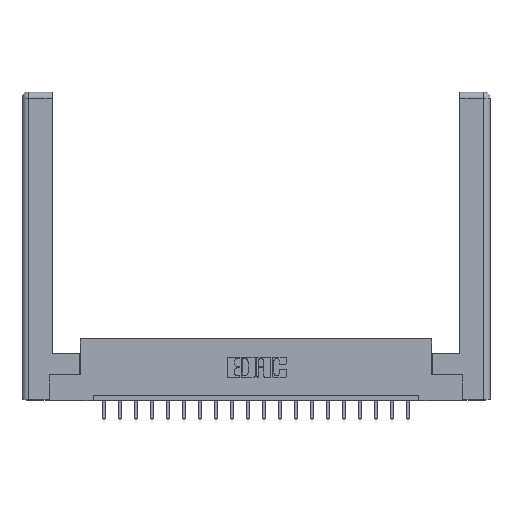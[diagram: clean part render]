
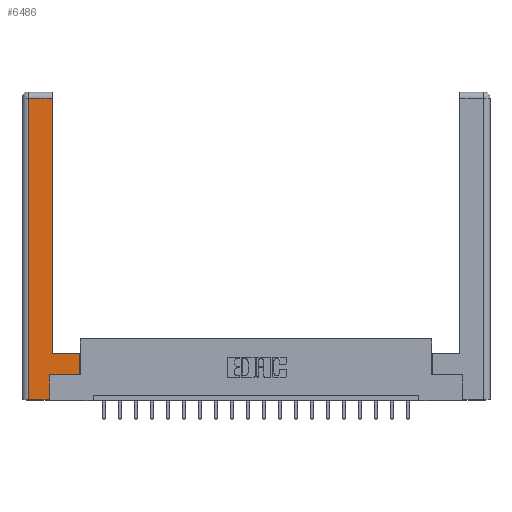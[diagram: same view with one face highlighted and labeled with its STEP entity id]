
A CAD part, top view. The second image highlights one B-rep face of the part: STEP entity #6486.
In plain terms, the highlighted planar face has unit normal (0, 0, 1).
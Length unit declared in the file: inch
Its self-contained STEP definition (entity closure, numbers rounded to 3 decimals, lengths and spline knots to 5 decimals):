
#60 = ORIENTED_EDGE ( 'NONE', *, *, #18326, .T. ) ;
#71 = PLANE ( 'NONE',  #1468 ) ;
#206 = ORIENTED_EDGE ( 'NONE', *, *, #640, .T. ) ;
#226 = DIRECTION ( 'NONE',  ( 0., -1., 0. ) ) ;
#282 = VECTOR ( 'NONE', #7637, 39.37008 ) ;
#640 = EDGE_CURVE ( 'NONE', #7224, #12169, #7378, .T. ) ;
#774 = CARTESIAN_POINT ( 'NONE',  ( 0.295, 2.94, 0. ) ) ;
#1060 = VERTEX_POINT ( 'NONE', #6679 ) ;
#1122 = VECTOR ( 'NONE', #226, 39.37008 ) ;
#1237 = CARTESIAN_POINT ( 'NONE',  ( 0.265, 0.245, 0. ) ) ;
#1468 = AXIS2_PLACEMENT_3D ( 'NONE', #14445, #1732, #1655 ) ;
#1655 = DIRECTION ( 'NONE',  ( -1., 0., 0. ) ) ;
#1732 = DIRECTION ( 'NONE',  ( 0., 0., -1. ) ) ;
#1901 = CARTESIAN_POINT ( 'NONE',  ( 0.565, 0.45, 0. ) ) ;
#1978 = EDGE_CURVE ( 'NONE', #12169, #1060, #11977, .T. ) ;
#2120 = LINE ( 'NONE', #3348, #1122 ) ;
#2153 = EDGE_CURVE ( 'NONE', #18739, #7224, #7045, .T. ) ;
#2240 = VERTEX_POINT ( 'NONE', #5527 ) ;
#2798 = VECTOR ( 'NONE', #3706, 39.37008 ) ;
#2805 = VECTOR ( 'NONE', #11432, 39.37008 ) ;
#3348 = CARTESIAN_POINT ( 'NONE',  ( 0.0615, 0., 0. ) ) ;
#3373 = ORIENTED_EDGE ( 'NONE', *, *, #14342, .T. ) ;
#3706 = DIRECTION ( 'NONE',  ( -1., 0., 0. ) ) ;
#3777 = LINE ( 'NONE', #5408, #11948 ) ;
#4193 = VERTEX_POINT ( 'NONE', #18626 ) ;
#4939 = EDGE_CURVE ( 'NONE', #2240, #4193, #10251, .T. ) ;
#5055 = VECTOR ( 'NONE', #6239, 39.37008 ) ;
#5352 = LINE ( 'NONE', #1901, #17923 ) ;
#5408 = CARTESIAN_POINT ( 'NONE',  ( 0.565, 0.245, 0. ) ) ;
#5441 = ORIENTED_EDGE ( 'NONE', *, *, #4939, .T. ) ;
#5527 = CARTESIAN_POINT ( 'NONE',  ( 0.0615, 0., 0. ) ) ;
#6239 = DIRECTION ( 'NONE',  ( -1., 0., 0. ) ) ;
#6486 = ADVANCED_FACE ( 'NONE', ( #15590 ), #71, .F. ) ;
#6679 = CARTESIAN_POINT ( 'NONE',  ( 0.0615, 2.94, 0. ) ) ;
#7045 = LINE ( 'NONE', #13186, #2798 ) ;
#7224 = VERTEX_POINT ( 'NONE', #16308 ) ;
#7378 = LINE ( 'NONE', #14216, #13511 ) ;
#7436 = CARTESIAN_POINT ( 'NONE',  ( 0.265, 0.245, 0. ) ) ;
#7622 = ORIENTED_EDGE ( 'NONE', *, *, #2153, .T. ) ;
#7637 = DIRECTION ( 'NONE',  ( 0., 1., 0. ) ) ;
#8750 = VERTEX_POINT ( 'NONE', #15575 ) ;
#10245 = ORIENTED_EDGE ( 'NONE', *, *, #14094, .T. ) ;
#10251 = LINE ( 'NONE', #14394, #2805 ) ;
#10887 = CARTESIAN_POINT ( 'NONE',  ( 0.0615, 2.94, 0. ) ) ;
#11432 = DIRECTION ( 'NONE',  ( 1., 0., 0. ) ) ;
#11702 = LINE ( 'NONE', #1237, #282 ) ;
#11948 = VECTOR ( 'NONE', #14651, 39.37008 ) ;
#11977 = LINE ( 'NONE', #10887, #5055 ) ;
#12102 = EDGE_LOOP ( 'NONE', ( #206, #17678, #60, #5441, #3373, #10245, #13100, #7622 ) ) ;
#12169 = VERTEX_POINT ( 'NONE', #774 ) ;
#12403 = CARTESIAN_POINT ( 'NONE',  ( 0.565, 0.45, 0. ) ) ;
#12642 = DIRECTION ( 'NONE',  ( 0., 1., 0. ) ) ;
#13100 = ORIENTED_EDGE ( 'NONE', *, *, #18277, .T. ) ;
#13186 = CARTESIAN_POINT ( 'NONE',  ( 0.295, 0.45, 0. ) ) ;
#13511 = VECTOR ( 'NONE', #12642, 39.37008 ) ;
#14094 = EDGE_CURVE ( 'NONE', #15529, #8750, #3777, .T. ) ;
#14216 = CARTESIAN_POINT ( 'NONE',  ( 0.295, 3., 0. ) ) ;
#14342 = EDGE_CURVE ( 'NONE', #4193, #15529, #11702, .T. ) ;
#14394 = CARTESIAN_POINT ( 'NONE',  ( 0.265, 0., 0. ) ) ;
#14445 = CARTESIAN_POINT ( 'NONE',  ( 0., 0., 0. ) ) ;
#14651 = DIRECTION ( 'NONE',  ( 1., 0., 0. ) ) ;
#15529 = VERTEX_POINT ( 'NONE', #7436 ) ;
#15575 = CARTESIAN_POINT ( 'NONE',  ( 0.565, 0.245, 0. ) ) ;
#15590 = FACE_OUTER_BOUND ( 'NONE', #12102, .T. ) ;
#15844 = DIRECTION ( 'NONE',  ( 0., 1., 0. ) ) ;
#16308 = CARTESIAN_POINT ( 'NONE',  ( 0.295, 0.45, 0. ) ) ;
#17678 = ORIENTED_EDGE ( 'NONE', *, *, #1978, .T. ) ;
#17923 = VECTOR ( 'NONE', #15844, 39.37008 ) ;
#18277 = EDGE_CURVE ( 'NONE', #8750, #18739, #5352, .T. ) ;
#18326 = EDGE_CURVE ( 'NONE', #1060, #2240, #2120, .T. ) ;
#18626 = CARTESIAN_POINT ( 'NONE',  ( 0.265, 0., 0. ) ) ;
#18739 = VERTEX_POINT ( 'NONE', #12403 ) ;
